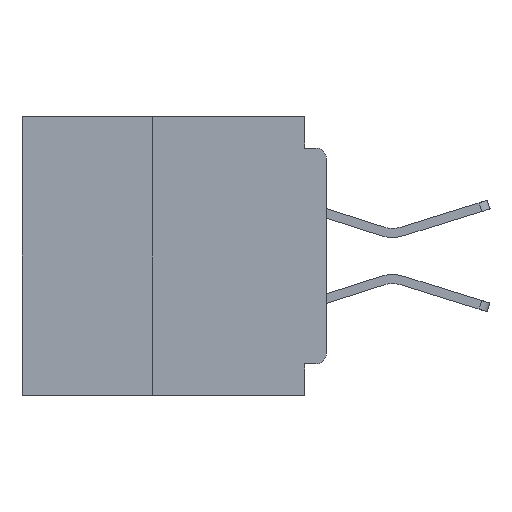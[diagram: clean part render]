
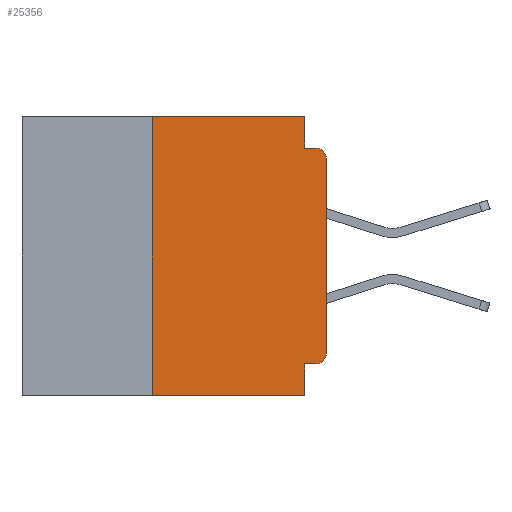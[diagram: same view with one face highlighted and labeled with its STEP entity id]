
A CAD part, left-side view. The second image highlights one B-rep face of the part: STEP entity #25356.
In plain terms, the highlighted planar face has unit normal (-1, 0, 0).
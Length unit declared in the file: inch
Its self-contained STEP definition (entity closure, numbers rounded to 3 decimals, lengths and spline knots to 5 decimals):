
#1113 = DIRECTION ( 'NONE',  ( 0., 0., 1. ) ) ;
#1372 = VECTOR ( 'NONE', #45475, 39.37008 ) ;
#1825 = CARTESIAN_POINT ( 'NONE',  ( 0., 0.031, -0.4 ) ) ;
#2061 = EDGE_CURVE ( 'NONE', #15952, #3792, #18350, .T. ) ;
#3037 = PLANE ( 'NONE',  #31270 ) ;
#3792 = VERTEX_POINT ( 'NONE', #32709 ) ;
#6246 = DIRECTION ( 'NONE',  ( 0., -1., 0. ) ) ;
#6683 = VECTOR ( 'NONE', #34946, 39.37008 ) ;
#6842 = DIRECTION ( 'NONE',  ( 0., 0., -1. ) ) ;
#7428 = VERTEX_POINT ( 'NONE', #7820 ) ;
#7820 = CARTESIAN_POINT ( 'NONE',  ( 0., 0., -0.06 ) ) ;
#8392 = LINE ( 'NONE', #47723, #27372 ) ;
#8450 = VERTEX_POINT ( 'NONE', #22119 ) ;
#8831 = CARTESIAN_POINT ( 'NONE',  ( 0., 0.015, -0.06 ) ) ;
#9139 = VERTEX_POINT ( 'NONE', #26025 ) ;
#10511 = CARTESIAN_POINT ( 'NONE',  ( 0., 0.437, 0. ) ) ;
#12660 = DIRECTION ( 'NONE',  ( 0., 0., -1. ) ) ;
#15952 = VERTEX_POINT ( 'NONE', #41111 ) ;
#18350 = LINE ( 'NONE', #26942, #47088 ) ;
#18691 = DIRECTION ( 'NONE',  ( 0., -1., 0. ) ) ;
#19242 = DIRECTION ( 'NONE',  ( -1., 0., 0. ) ) ;
#19789 = CARTESIAN_POINT ( 'NONE',  ( 0., 0., -0.355 ) ) ;
#19831 = LINE ( 'NONE', #48494, #47381 ) ;
#20069 = ORIENTED_EDGE ( 'NONE', *, *, #41092, .T. ) ;
#20637 = ORIENTED_EDGE ( 'NONE', *, *, #21237, .T. ) ;
#21237 = EDGE_CURVE ( 'NONE', #28710, #7428, #24875, .T. ) ;
#21498 = VERTEX_POINT ( 'NONE', #44160 ) ;
#22046 = VERTEX_POINT ( 'NONE', #36323 ) ;
#22119 = CARTESIAN_POINT ( 'NONE',  ( 0., 0.031, -0.4 ) ) ;
#22211 = CARTESIAN_POINT ( 'NONE',  ( 0., 0., -0.34 ) ) ;
#23004 = CARTESIAN_POINT ( 'NONE',  ( 0., 0.437, 0. ) ) ;
#24218 = VECTOR ( 'NONE', #32154, 39.37008 ) ;
#24875 = LINE ( 'NONE', #35209, #34908 ) ;
#24959 = CARTESIAN_POINT ( 'NONE',  ( 0., 0.015, -0.355 ) ) ;
#25017 = ORIENTED_EDGE ( 'NONE', *, *, #31665, .F. ) ;
#25356 = ADVANCED_FACE ( 'NONE', ( #38142 ), #3037, .F. ) ;
#25557 = DIRECTION ( 'NONE',  ( 0., 0., 1. ) ) ;
#26025 = CARTESIAN_POINT ( 'NONE',  ( 0., 0.031, -0.355 ) ) ;
#26655 = ORIENTED_EDGE ( 'NONE', *, *, #30956, .T. ) ;
#26859 = LINE ( 'NONE', #19789, #6683 ) ;
#26942 = CARTESIAN_POINT ( 'NONE',  ( 0., 0.031, 0. ) ) ;
#27372 = VECTOR ( 'NONE', #6246, 39.37008 ) ;
#27734 = CIRCLE ( 'NONE', #28138, 0.015 ) ;
#28138 = AXIS2_PLACEMENT_3D ( 'NONE', #8831, #35301, #12660 ) ;
#28441 = EDGE_CURVE ( 'NONE', #9139, #8450, #44186, .T. ) ;
#28710 = VERTEX_POINT ( 'NONE', #22211 ) ;
#29554 = DIRECTION ( 'NONE',  ( 1., 0., 0. ) ) ;
#30377 = EDGE_CURVE ( 'NONE', #40354, #28710, #45723, .T. ) ;
#30956 = EDGE_CURVE ( 'NONE', #44007, #8450, #19831, .T. ) ;
#31148 = ORIENTED_EDGE ( 'NONE', *, *, #2061, .F. ) ;
#31270 = AXIS2_PLACEMENT_3D ( 'NONE', #10511, #29554, #6842 ) ;
#31665 = EDGE_CURVE ( 'NONE', #40354, #9139, #26859, .T. ) ;
#32154 = DIRECTION ( 'NONE',  ( 0., 0., -1. ) ) ;
#32312 = EDGE_CURVE ( 'NONE', #3792, #22046, #8392, .T. ) ;
#32709 = CARTESIAN_POINT ( 'NONE',  ( 0., 0.031, -0.045 ) ) ;
#32780 = EDGE_LOOP ( 'NONE', ( #20637, #20069, #44733, #31148, #36627, #44431, #26655, #48047, #25017, #43955 ) ) ;
#33471 = EDGE_CURVE ( 'NONE', #44007, #21498, #46724, .T. ) ;
#34908 = VECTOR ( 'NONE', #1113, 39.37008 ) ;
#34946 = DIRECTION ( 'NONE',  ( 0., 1., 0. ) ) ;
#35209 = CARTESIAN_POINT ( 'NONE',  ( 0., 0., 0. ) ) ;
#35301 = DIRECTION ( 'NONE',  ( -1., 0., 0. ) ) ;
#36323 = CARTESIAN_POINT ( 'NONE',  ( 0., 0.015, -0.045 ) ) ;
#36627 = ORIENTED_EDGE ( 'NONE', *, *, #43423, .F. ) ;
#36895 = VECTOR ( 'NONE', #25557, 39.37008 ) ;
#38092 = AXIS2_PLACEMENT_3D ( 'NONE', #41773, #19242, #45491 ) ;
#38142 = FACE_OUTER_BOUND ( 'NONE', #32780, .T. ) ;
#40354 = VERTEX_POINT ( 'NONE', #24959 ) ;
#41092 = EDGE_CURVE ( 'NONE', #7428, #22046, #27734, .T. ) ;
#41111 = CARTESIAN_POINT ( 'NONE',  ( 0., 0.031, 0. ) ) ;
#41711 = CARTESIAN_POINT ( 'NONE',  ( 0., 0.25, -0.4 ) ) ;
#41773 = CARTESIAN_POINT ( 'NONE',  ( 0., 0.015, -0.34 ) ) ;
#42736 = LINE ( 'NONE', #23004, #1372 ) ;
#43423 = EDGE_CURVE ( 'NONE', #21498, #15952, #42736, .T. ) ;
#43955 = ORIENTED_EDGE ( 'NONE', *, *, #30377, .T. ) ;
#44007 = VERTEX_POINT ( 'NONE', #41711 ) ;
#44160 = CARTESIAN_POINT ( 'NONE',  ( 0., 0.25, 0. ) ) ;
#44186 = LINE ( 'NONE', #1825, #24218 ) ;
#44256 = CARTESIAN_POINT ( 'NONE',  ( 0., 0.25, -0.4 ) ) ;
#44431 = ORIENTED_EDGE ( 'NONE', *, *, #33471, .F. ) ;
#44733 = ORIENTED_EDGE ( 'NONE', *, *, #32312, .F. ) ;
#45475 = DIRECTION ( 'NONE',  ( 0., -1., 0. ) ) ;
#45491 = DIRECTION ( 'NONE',  ( 0., 0., -1. ) ) ;
#45723 = CIRCLE ( 'NONE', #38092, 0.015 ) ;
#46724 = LINE ( 'NONE', #44256, #36895 ) ;
#46824 = DIRECTION ( 'NONE',  ( 0., 0., -1. ) ) ;
#47088 = VECTOR ( 'NONE', #46824, 39.37008 ) ;
#47381 = VECTOR ( 'NONE', #18691, 39.37008 ) ;
#47723 = CARTESIAN_POINT ( 'NONE',  ( 0., 0., -0.045 ) ) ;
#48047 = ORIENTED_EDGE ( 'NONE', *, *, #28441, .F. ) ;
#48494 = CARTESIAN_POINT ( 'NONE',  ( 0., 0.437, -0.4 ) ) ;
